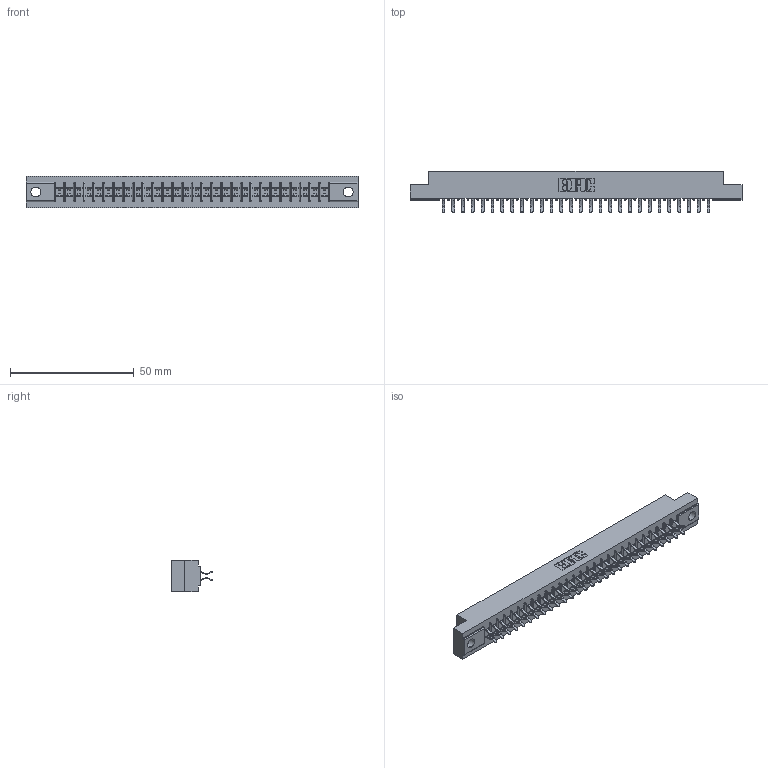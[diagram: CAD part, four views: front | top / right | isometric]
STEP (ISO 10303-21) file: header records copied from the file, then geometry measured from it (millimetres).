
FILE_DESCRIPTION (( 'STEP AP203' ), '1' );
FILE_NAME ('315-056-556-204.STEP', '2019-09-10T19:33:31', ( '' ), ( '' ), 'SwSTEP 2.0', 'SolidWorks 2016', '' );
FILE_SCHEMA (( 'CONFIG_CONTROL_DESIGN' ));
Length unit declared in the file: inch
Products named in the file (3): 305 Part_.156 Dia; 305-290-001_556; 315-056-556-204
Assembly tree (57 placements, depth 2):
  315-056-556-204
    305 Part_.156 Dia
    305-290-001_556  x56
Bounding box: 133.96 x 16.64 x 12.7 mm (x, y, z)
Volume: 13780.9 mm3; surface area: 17058.6 mm2
Topology: 57 solids, 57 shells, 3266 faces, 9396 edges, 6112 vertices
Faces by surface type: plane 1818, cylinder 1336, sphere 112
Entity records: 32661 total; most frequent: CARTESIAN_POINT 5412, ORIENTED_EDGE 5368, DIRECTION 5242, EDGE_CURVE 2684, LINE 2158, VECTOR 2158, VERTEX_POINT 1712, AXIS2_PLACEMENT_3D 1542
